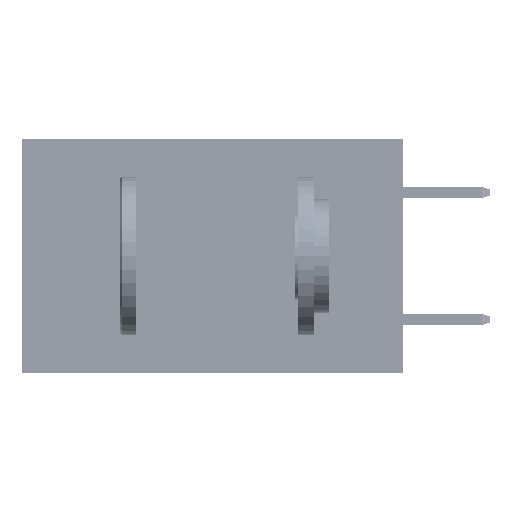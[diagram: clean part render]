
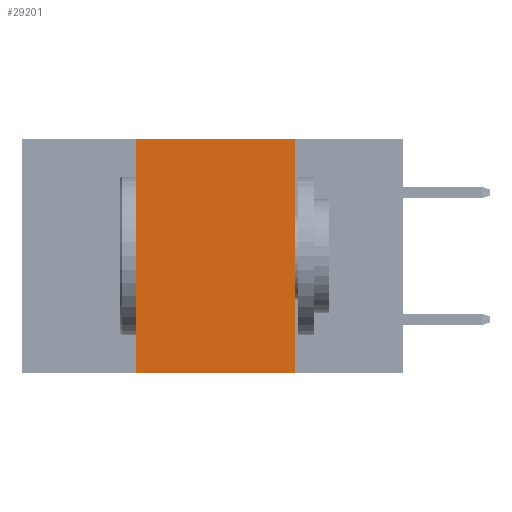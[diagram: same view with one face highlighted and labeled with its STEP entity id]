
A CAD part, left-side view. The second image highlights one B-rep face of the part: STEP entity #29201.
In plain terms, the highlighted planar face has unit normal (-1, 0, 0).
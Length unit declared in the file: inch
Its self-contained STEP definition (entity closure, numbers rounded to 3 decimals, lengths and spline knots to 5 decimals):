
#1696 = EDGE_LOOP ( 'NONE', ( #40149, #34181, #20268, #4003 ) ) ;
#4003 = ORIENTED_EDGE ( 'NONE', *, *, #49727, .T. ) ;
#6188 = FACE_OUTER_BOUND ( 'NONE', #1696, .T. ) ;
#6281 = CARTESIAN_POINT ( 'NONE',  ( 0., 0.17, 0. ) ) ;
#10710 = DIRECTION ( 'NONE',  ( 1., 0., 0. ) ) ;
#15628 = CARTESIAN_POINT ( 'NONE',  ( 0., 0.42, -0.37 ) ) ;
#16366 = EDGE_CURVE ( 'NONE', #41758, #19919, #32318, .T. ) ;
#16625 = AXIS2_PLACEMENT_3D ( 'NONE', #47280, #10710, #47021 ) ;
#19719 = LINE ( 'NONE', #23991, #20138 ) ;
#19919 = VERTEX_POINT ( 'NONE', #22644 ) ;
#20138 = VECTOR ( 'NONE', #23733, 39.37008 ) ;
#20268 = ORIENTED_EDGE ( 'NONE', *, *, #45523, .F. ) ;
#22644 = CARTESIAN_POINT ( 'NONE',  ( 0., 0.17, -0.37 ) ) ;
#23733 = DIRECTION ( 'NONE',  ( 0., 0., 1. ) ) ;
#23991 = CARTESIAN_POINT ( 'NONE',  ( 0., 0.42, 0. ) ) ;
#26900 = VECTOR ( 'NONE', #32837, 39.37008 ) ;
#29201 = ADVANCED_FACE ( 'NONE', ( #6188 ), #30740, .F. ) ;
#30603 = CARTESIAN_POINT ( 'NONE',  ( 0., 0.42, 0. ) ) ;
#30740 = PLANE ( 'NONE',  #16625 ) ;
#31920 = DIRECTION ( 'NONE',  ( 0., -1., 0. ) ) ;
#32318 = LINE ( 'NONE', #48596, #26900 ) ;
#32837 = DIRECTION ( 'NONE',  ( 0., 0., -1. ) ) ;
#34181 = ORIENTED_EDGE ( 'NONE', *, *, #46000, .F. ) ;
#36976 = CARTESIAN_POINT ( 'NONE',  ( 0., 0.6, 0. ) ) ;
#38700 = VERTEX_POINT ( 'NONE', #30603 ) ;
#40149 = ORIENTED_EDGE ( 'NONE', *, *, #16366, .F. ) ;
#41389 = DIRECTION ( 'NONE',  ( 0., -1., 0. ) ) ;
#41758 = VERTEX_POINT ( 'NONE', #6281 ) ;
#44600 = LINE ( 'NONE', #44872, #52645 ) ;
#44872 = CARTESIAN_POINT ( 'NONE',  ( 0., 0.6, -0.37 ) ) ;
#45523 = EDGE_CURVE ( 'NONE', #50748, #38700, #19719, .T. ) ;
#46000 = EDGE_CURVE ( 'NONE', #38700, #41758, #47943, .T. ) ;
#47021 = DIRECTION ( 'NONE',  ( 0., 0., -1. ) ) ;
#47280 = CARTESIAN_POINT ( 'NONE',  ( 0., 0.6, 0. ) ) ;
#47943 = LINE ( 'NONE', #36976, #52512 ) ;
#48596 = CARTESIAN_POINT ( 'NONE',  ( 0., 0.17, 0. ) ) ;
#49727 = EDGE_CURVE ( 'NONE', #50748, #19919, #44600, .T. ) ;
#50748 = VERTEX_POINT ( 'NONE', #15628 ) ;
#52512 = VECTOR ( 'NONE', #31920, 39.37008 ) ;
#52645 = VECTOR ( 'NONE', #41389, 39.37008 ) ;
